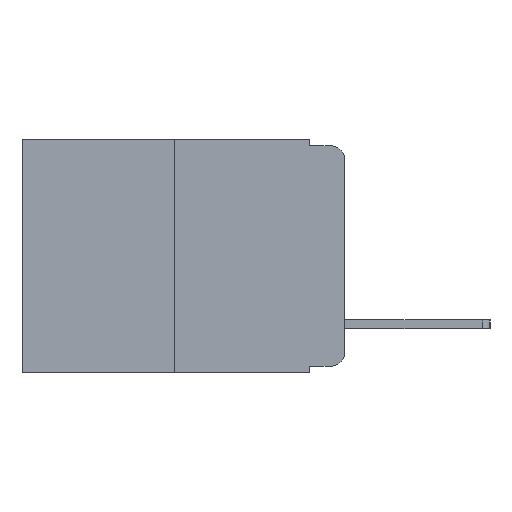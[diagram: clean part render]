
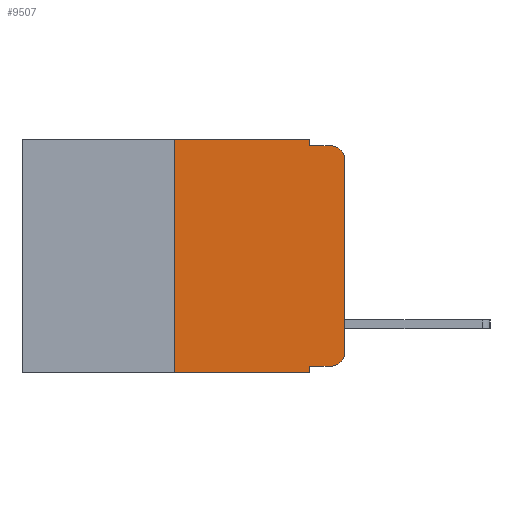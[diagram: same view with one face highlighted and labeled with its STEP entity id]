
A CAD part, left-side view. The second image highlights one B-rep face of the part: STEP entity #9507.
In plain terms, the highlighted planar face has unit normal (-1, 0, 0).
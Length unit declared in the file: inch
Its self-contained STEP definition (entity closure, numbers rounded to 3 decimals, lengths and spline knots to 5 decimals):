
#333 = VECTOR ( 'NONE', #9168, 39.37008 ) ;
#440 = ORIENTED_EDGE ( 'NONE', *, *, #17096, .F. ) ;
#850 = CARTESIAN_POINT ( 'NONE',  ( 0., 0.25, -0.343 ) ) ;
#898 = LINE ( 'NONE', #4204, #333 ) ;
#1138 = VERTEX_POINT ( 'NONE', #18277 ) ;
#1289 = VERTEX_POINT ( 'NONE', #17234 ) ;
#1370 = CARTESIAN_POINT ( 'NONE',  ( 0., 0., -0.313 ) ) ;
#1539 = CARTESIAN_POINT ( 'NONE',  ( 0., 0.02, -0.313 ) ) ;
#1652 = VERTEX_POINT ( 'NONE', #13696 ) ;
#1718 = VERTEX_POINT ( 'NONE', #850 ) ;
#2564 = DIRECTION ( 'NONE',  ( 0., 0., 1. ) ) ;
#3213 = CARTESIAN_POINT ( 'NONE',  ( 0., 0.02, -0.03 ) ) ;
#3341 = DIRECTION ( 'NONE',  ( 0., 0., -1. ) ) ;
#4204 = CARTESIAN_POINT ( 'NONE',  ( 0., 0., 0. ) ) ;
#4456 = DIRECTION ( 'NONE',  ( 0., -1., 0. ) ) ;
#4611 = EDGE_CURVE ( 'NONE', #1289, #14226, #9350, .T. ) ;
#4829 = LINE ( 'NONE', #16859, #17023 ) ;
#4856 = DIRECTION ( 'NONE',  ( 0., 0., -1. ) ) ;
#5020 = ORIENTED_EDGE ( 'NONE', *, *, #10622, .T. ) ;
#5751 = VECTOR ( 'NONE', #6389, 39.37008 ) ;
#5896 = CARTESIAN_POINT ( 'NONE',  ( 0., 0.051, 0. ) ) ;
#5946 = EDGE_CURVE ( 'NONE', #14226, #7950, #898, .T. ) ;
#6053 = VERTEX_POINT ( 'NONE', #17542 ) ;
#6318 = ORIENTED_EDGE ( 'NONE', *, *, #18773, .T. ) ;
#6389 = DIRECTION ( 'NONE',  ( 0., -1., 0. ) ) ;
#7020 = PLANE ( 'NONE',  #17832 ) ;
#7437 = DIRECTION ( 'NONE',  ( 0., -1., 0. ) ) ;
#7562 = CARTESIAN_POINT ( 'NONE',  ( 0., 0.051, -0.01 ) ) ;
#7950 = VERTEX_POINT ( 'NONE', #15147 ) ;
#8008 = EDGE_CURVE ( 'NONE', #17934, #1652, #4829, .T. ) ;
#8213 = VECTOR ( 'NONE', #20625, 39.37008 ) ;
#8609 = CIRCLE ( 'NONE', #17808, 0.02 ) ;
#8853 = LINE ( 'NONE', #5896, #20704 ) ;
#9168 = DIRECTION ( 'NONE',  ( 0., 0., 1. ) ) ;
#9350 = CIRCLE ( 'NONE', #15963, 0.02 ) ;
#9358 = VECTOR ( 'NONE', #4456, 39.37008 ) ;
#9507 = ADVANCED_FACE ( 'NONE', ( #14833 ), #7020, .F. ) ;
#9596 = LINE ( 'NONE', #15900, #5751 ) ;
#9886 = ORIENTED_EDGE ( 'NONE', *, *, #12506, .F. ) ;
#10136 = EDGE_CURVE ( 'NONE', #17601, #17934, #8853, .T. ) ;
#10518 = EDGE_CURVE ( 'NONE', #12990, #1289, #16684, .T. ) ;
#10622 = EDGE_CURVE ( 'NONE', #1718, #1138, #9596, .T. ) ;
#10857 = LINE ( 'NONE', #19998, #14538 ) ;
#11666 = ORIENTED_EDGE ( 'NONE', *, *, #8008, .F. ) ;
#11837 = LINE ( 'NONE', #15083, #15482 ) ;
#12506 = EDGE_CURVE ( 'NONE', #12990, #1138, #12528, .T. ) ;
#12528 = LINE ( 'NONE', #17529, #8213 ) ;
#12574 = CARTESIAN_POINT ( 'NONE',  ( 0., 0.051, -0.333 ) ) ;
#12990 = VERTEX_POINT ( 'NONE', #20817 ) ;
#13072 = DIRECTION ( 'NONE',  ( -1., 0., 0. ) ) ;
#13142 = ORIENTED_EDGE ( 'NONE', *, *, #19800, .F. ) ;
#13409 = DIRECTION ( 'NONE',  ( 1., 0., 0. ) ) ;
#13696 = CARTESIAN_POINT ( 'NONE',  ( 0., 0.02, -0.01 ) ) ;
#13889 = ORIENTED_EDGE ( 'NONE', *, *, #5946, .T. ) ;
#14226 = VERTEX_POINT ( 'NONE', #1370 ) ;
#14524 = DIRECTION ( 'NONE',  ( -1., 0., 0. ) ) ;
#14538 = VECTOR ( 'NONE', #2564, 39.37008 ) ;
#14557 = DIRECTION ( 'NONE',  ( 0., 0., -1. ) ) ;
#14833 = FACE_OUTER_BOUND ( 'NONE', #18397, .T. ) ;
#14947 = CARTESIAN_POINT ( 'NONE',  ( 0., 0.473, 0. ) ) ;
#15083 = CARTESIAN_POINT ( 'NONE',  ( 0., 0.473, 0. ) ) ;
#15147 = CARTESIAN_POINT ( 'NONE',  ( 0., 0., -0.03 ) ) ;
#15482 = VECTOR ( 'NONE', #19651, 39.37008 ) ;
#15900 = CARTESIAN_POINT ( 'NONE',  ( 0., 0.473, -0.343 ) ) ;
#15963 = AXIS2_PLACEMENT_3D ( 'NONE', #1539, #13072, #3341 ) ;
#16684 = LINE ( 'NONE', #12574, #9358 ) ;
#16728 = ORIENTED_EDGE ( 'NONE', *, *, #10136, .F. ) ;
#16859 = CARTESIAN_POINT ( 'NONE',  ( 0., 0.051, -0.01 ) ) ;
#17023 = VECTOR ( 'NONE', #7437, 39.37008 ) ;
#17096 = EDGE_CURVE ( 'NONE', #1718, #6053, #10857, .T. ) ;
#17234 = CARTESIAN_POINT ( 'NONE',  ( 0., 0.02, -0.333 ) ) ;
#17529 = CARTESIAN_POINT ( 'NONE',  ( 0., 0.051, 0. ) ) ;
#17542 = CARTESIAN_POINT ( 'NONE',  ( 0., 0.25, 0. ) ) ;
#17601 = VERTEX_POINT ( 'NONE', #17924 ) ;
#17808 = AXIS2_PLACEMENT_3D ( 'NONE', #3213, #14524, #4856 ) ;
#17832 = AXIS2_PLACEMENT_3D ( 'NONE', #14947, #13409, #18001 ) ;
#17924 = CARTESIAN_POINT ( 'NONE',  ( 0., 0.051, 0. ) ) ;
#17934 = VERTEX_POINT ( 'NONE', #7562 ) ;
#18001 = DIRECTION ( 'NONE',  ( 0., 0., -1. ) ) ;
#18164 = ORIENTED_EDGE ( 'NONE', *, *, #10518, .T. ) ;
#18277 = CARTESIAN_POINT ( 'NONE',  ( 0., 0.051, -0.343 ) ) ;
#18397 = EDGE_LOOP ( 'NONE', ( #13889, #6318, #11666, #16728, #13142, #440, #5020, #9886, #18164, #19113 ) ) ;
#18773 = EDGE_CURVE ( 'NONE', #7950, #1652, #8609, .T. ) ;
#19113 = ORIENTED_EDGE ( 'NONE', *, *, #4611, .T. ) ;
#19651 = DIRECTION ( 'NONE',  ( 0., -1., 0. ) ) ;
#19800 = EDGE_CURVE ( 'NONE', #6053, #17601, #11837, .T. ) ;
#19998 = CARTESIAN_POINT ( 'NONE',  ( 0., 0.25, 0. ) ) ;
#20625 = DIRECTION ( 'NONE',  ( 0., 0., -1. ) ) ;
#20704 = VECTOR ( 'NONE', #14557, 39.37008 ) ;
#20817 = CARTESIAN_POINT ( 'NONE',  ( 0., 0.051, -0.333 ) ) ;
